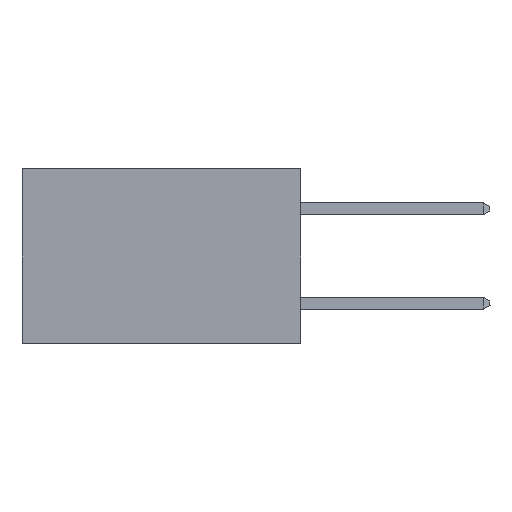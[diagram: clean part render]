
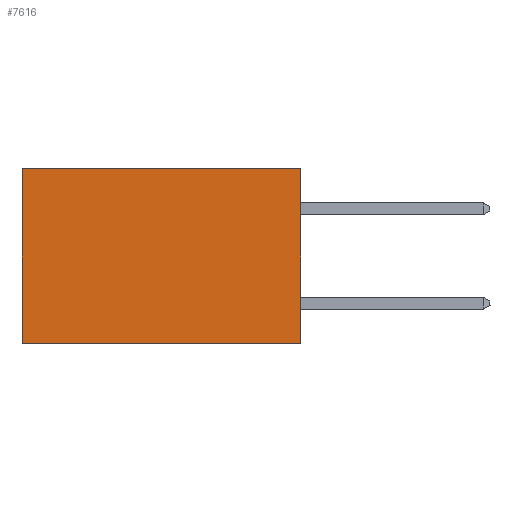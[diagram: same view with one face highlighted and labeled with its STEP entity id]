
A CAD part, left-side view. The second image highlights one B-rep face of the part: STEP entity #7616.
In plain terms, the highlighted planar face has unit normal (-1, 0, 0).
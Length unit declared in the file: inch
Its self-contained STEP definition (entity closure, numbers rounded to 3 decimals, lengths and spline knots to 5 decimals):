
#1228 = VECTOR ( 'NONE', #3400, 39.37008 ) ;
#1457 = EDGE_CURVE ( 'NONE', #10704, #7668, #14500, .T. ) ;
#1912 = ORIENTED_EDGE ( 'NONE', *, *, #10591, .F. ) ;
#2270 = AXIS2_PLACEMENT_3D ( 'NONE', #18212, #3305, #14942 ) ;
#2437 = VERTEX_POINT ( 'NONE', #3881 ) ;
#3305 = DIRECTION ( 'NONE',  ( 1., 0., 0. ) ) ;
#3400 = DIRECTION ( 'NONE',  ( 0., 1., 0. ) ) ;
#3444 = CARTESIAN_POINT ( 'NONE',  ( 0.277, 0.59, -0.37 ) ) ;
#3860 = CARTESIAN_POINT ( 'NONE',  ( 0.277, 0., -0.37 ) ) ;
#3881 = CARTESIAN_POINT ( 'NONE',  ( 0.277, 0.59, 0. ) ) ;
#4462 = CARTESIAN_POINT ( 'NONE',  ( 0.277, 0., 0. ) ) ;
#5641 = ORIENTED_EDGE ( 'NONE', *, *, #1457, .F. ) ;
#5932 = CARTESIAN_POINT ( 'NONE',  ( 0.277, 0.59, -0.37 ) ) ;
#6045 = ORIENTED_EDGE ( 'NONE', *, *, #18060, .T. ) ;
#6148 = DIRECTION ( 'NONE',  ( 0., 1., 0. ) ) ;
#7242 = VECTOR ( 'NONE', #21436, 39.37008 ) ;
#7616 = ADVANCED_FACE ( 'NONE', ( #16106 ), #13308, .F. ) ;
#7668 = VERTEX_POINT ( 'NONE', #3444 ) ;
#8490 = LINE ( 'NONE', #5932, #16763 ) ;
#9712 = LINE ( 'NONE', #4462, #17999 ) ;
#9877 = CARTESIAN_POINT ( 'NONE',  ( 0.277, 0., -0.37 ) ) ;
#10591 = EDGE_CURVE ( 'NONE', #10824, #10704, #19427, .T. ) ;
#10704 = VERTEX_POINT ( 'NONE', #18338 ) ;
#10824 = VERTEX_POINT ( 'NONE', #20297 ) ;
#11604 = EDGE_LOOP ( 'NONE', ( #6045, #5641, #1912, #20683 ) ) ;
#13308 = PLANE ( 'NONE',  #2270 ) ;
#13455 = EDGE_CURVE ( 'NONE', #10824, #2437, #9712, .T. ) ;
#14500 = LINE ( 'NONE', #3860, #1228 ) ;
#14942 = DIRECTION ( 'NONE',  ( 0., 0., -1. ) ) ;
#15875 = DIRECTION ( 'NONE',  ( 0., 0., -1. ) ) ;
#16106 = FACE_OUTER_BOUND ( 'NONE', #11604, .T. ) ;
#16763 = VECTOR ( 'NONE', #15875, 39.37008 ) ;
#17999 = VECTOR ( 'NONE', #6148, 39.37008 ) ;
#18060 = EDGE_CURVE ( 'NONE', #2437, #7668, #8490, .T. ) ;
#18212 = CARTESIAN_POINT ( 'NONE',  ( 0.277, 0., -0.37 ) ) ;
#18338 = CARTESIAN_POINT ( 'NONE',  ( 0.277, 0., -0.37 ) ) ;
#19427 = LINE ( 'NONE', #9877, #7242 ) ;
#20297 = CARTESIAN_POINT ( 'NONE',  ( 0.277, 0., 0. ) ) ;
#20683 = ORIENTED_EDGE ( 'NONE', *, *, #13455, .T. ) ;
#21436 = DIRECTION ( 'NONE',  ( 0., 0., -1. ) ) ;
